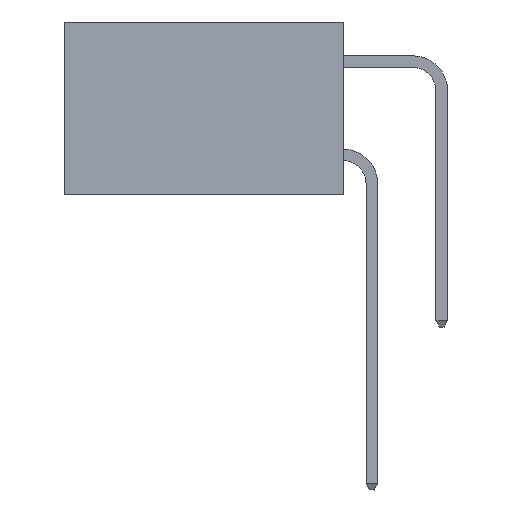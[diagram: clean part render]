
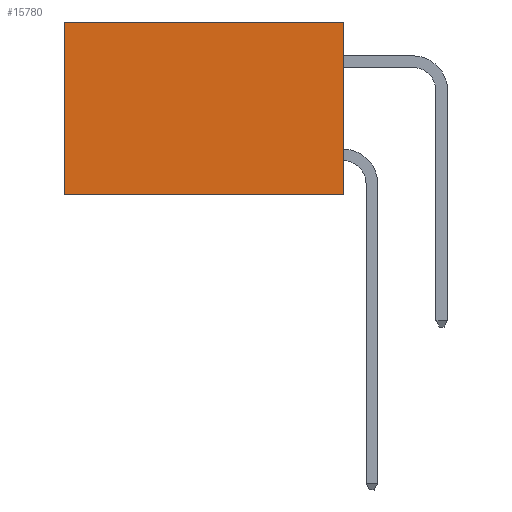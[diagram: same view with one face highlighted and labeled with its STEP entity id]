
A CAD part, left-side view. The second image highlights one B-rep face of the part: STEP entity #15780.
In plain terms, the highlighted planar face has unit normal (-1, 0, 0).
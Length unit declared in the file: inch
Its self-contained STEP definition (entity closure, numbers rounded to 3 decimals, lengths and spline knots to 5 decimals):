
#25 = VERTEX_POINT ( 'NONE', #1941 ) ;
#1941 = CARTESIAN_POINT ( 'NONE',  ( 0.2615, 0., -0.37 ) ) ;
#2089 = FACE_OUTER_BOUND ( 'NONE', #17167, .T. ) ;
#2682 = VECTOR ( 'NONE', #17060, 39.37008 ) ;
#3172 = CARTESIAN_POINT ( 'NONE',  ( 0.2615, 0., 0. ) ) ;
#3590 = PLANE ( 'NONE',  #18494 ) ;
#5662 = CARTESIAN_POINT ( 'NONE',  ( 0.2615, 0., -0.37 ) ) ;
#6462 = CARTESIAN_POINT ( 'NONE',  ( 0.2615, 0., 0. ) ) ;
#7083 = CARTESIAN_POINT ( 'NONE',  ( 0.2615, 0., -0.37 ) ) ;
#7195 = LINE ( 'NONE', #7083, #21498 ) ;
#7327 = VECTOR ( 'NONE', #10018, 39.37008 ) ;
#7940 = ORIENTED_EDGE ( 'NONE', *, *, #15407, .F. ) ;
#7998 = LINE ( 'NONE', #19776, #11804 ) ;
#8189 = VERTEX_POINT ( 'NONE', #19585 ) ;
#8287 = CARTESIAN_POINT ( 'NONE',  ( 0.2615, 0., -0.37 ) ) ;
#9476 = ORIENTED_EDGE ( 'NONE', *, *, #13444, .T. ) ;
#9733 = DIRECTION ( 'NONE',  ( 0., 0., -1. ) ) ;
#9968 = LINE ( 'NONE', #3172, #2682 ) ;
#10018 = DIRECTION ( 'NONE',  ( 0., 0., -1. ) ) ;
#10626 = DIRECTION ( 'NONE',  ( 0., 0., -1. ) ) ;
#11804 = VECTOR ( 'NONE', #9733, 39.37008 ) ;
#13444 = EDGE_CURVE ( 'NONE', #14111, #8189, #7998, .T. ) ;
#14111 = VERTEX_POINT ( 'NONE', #20977 ) ;
#14184 = EDGE_CURVE ( 'NONE', #20798, #25, #20249, .T. ) ;
#14248 = DIRECTION ( 'NONE',  ( 0., 1., 0. ) ) ;
#15407 = EDGE_CURVE ( 'NONE', #25, #8189, #7195, .T. ) ;
#15780 = ADVANCED_FACE ( 'NONE', ( #2089 ), #3590, .F. ) ;
#16578 = ORIENTED_EDGE ( 'NONE', *, *, #14184, .F. ) ;
#17060 = DIRECTION ( 'NONE',  ( 0., 1., 0. ) ) ;
#17167 = EDGE_LOOP ( 'NONE', ( #9476, #7940, #16578, #19271 ) ) ;
#18187 = EDGE_CURVE ( 'NONE', #20798, #14111, #9968, .T. ) ;
#18494 = AXIS2_PLACEMENT_3D ( 'NONE', #5662, #19581, #10626 ) ;
#19271 = ORIENTED_EDGE ( 'NONE', *, *, #18187, .T. ) ;
#19581 = DIRECTION ( 'NONE',  ( 1., 0., 0. ) ) ;
#19585 = CARTESIAN_POINT ( 'NONE',  ( 0.2615, 0.6, -0.37 ) ) ;
#19776 = CARTESIAN_POINT ( 'NONE',  ( 0.2615, 0.6, -0.37 ) ) ;
#20249 = LINE ( 'NONE', #8287, #7327 ) ;
#20798 = VERTEX_POINT ( 'NONE', #6462 ) ;
#20977 = CARTESIAN_POINT ( 'NONE',  ( 0.2615, 0.6, 0. ) ) ;
#21498 = VECTOR ( 'NONE', #14248, 39.37008 ) ;
